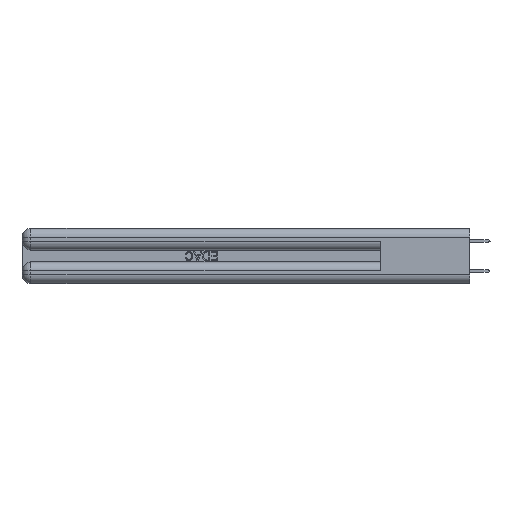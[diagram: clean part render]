
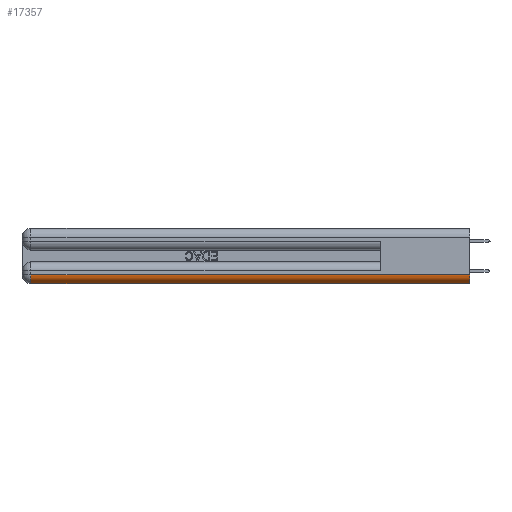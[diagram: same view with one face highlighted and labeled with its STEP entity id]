
A CAD part, left-side view. The second image highlights one B-rep face of the part: STEP entity #17357.
In plain terms, the highlighted cylindrical face has radius 1.524 mm (diameter 3.048 mm), a partial arc.
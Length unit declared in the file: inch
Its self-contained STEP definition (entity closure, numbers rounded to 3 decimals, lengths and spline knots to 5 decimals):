
#22 = CYLINDRICAL_SURFACE ( 'NONE', #30454, 0.06 ) ;
#61 = LINE ( 'NONE', #21087, #33446 ) ;
#102 = AXIS2_PLACEMENT_3D ( 'NONE', #38041, #6338, #45250 ) ;
#2767 = VERTEX_POINT ( 'NONE', #3020 ) ;
#3020 = CARTESIAN_POINT ( 'NONE',  ( 0., 0., 0.06 ) ) ;
#3803 = DIRECTION ( 'NONE',  ( 0., -1., 0. ) ) ;
#6338 = DIRECTION ( 'NONE',  ( 0., 1., 0. ) ) ;
#7774 = CARTESIAN_POINT ( 'NONE',  ( 0.06, 2.94, 0. ) ) ;
#9703 = DIRECTION ( 'NONE',  ( 0., -1., 0. ) ) ;
#9736 = CIRCLE ( 'NONE', #102, 0.06 ) ;
#13907 = DIRECTION ( 'NONE',  ( 0., 0., 1. ) ) ;
#17357 = ADVANCED_FACE ( 'NONE', ( #35016 ), #22, .T. ) ;
#20125 = EDGE_CURVE ( 'NONE', #2767, #30517, #38081, .T. ) ;
#21087 = CARTESIAN_POINT ( 'NONE',  ( 0., 0., 0.06 ) ) ;
#21314 = CARTESIAN_POINT ( 'NONE',  ( 0., 2.94, 0.06 ) ) ;
#23060 = ORIENTED_EDGE ( 'NONE', *, *, #20125, .F. ) ;
#23901 = AXIS2_PLACEMENT_3D ( 'NONE', #42094, #9703, #13907 ) ;
#24977 = CARTESIAN_POINT ( 'NONE',  ( 0.06, 0., 0.06 ) ) ;
#29100 = CARTESIAN_POINT ( 'NONE',  ( 0.06, 0., 0. ) ) ;
#29846 = LINE ( 'NONE', #33559, #37324 ) ;
#30108 = EDGE_CURVE ( 'NONE', #43690, #2767, #61, .T. ) ;
#30454 = AXIS2_PLACEMENT_3D ( 'NONE', #24977, #42917, #31294 ) ;
#30517 = VERTEX_POINT ( 'NONE', #29100 ) ;
#31294 = DIRECTION ( 'NONE',  ( 0., 0., 1. ) ) ;
#31676 = EDGE_CURVE ( 'NONE', #32683, #43690, #9736, .T. ) ;
#31898 = EDGE_CURVE ( 'NONE', #30517, #32683, #29846, .T. ) ;
#32683 = VERTEX_POINT ( 'NONE', #7774 ) ;
#33446 = VECTOR ( 'NONE', #3803, 39.37008 ) ;
#33559 = CARTESIAN_POINT ( 'NONE',  ( 0.06, 3., 0. ) ) ;
#35016 = FACE_OUTER_BOUND ( 'NONE', #36921, .T. ) ;
#35909 = ORIENTED_EDGE ( 'NONE', *, *, #31898, .F. ) ;
#36375 = DIRECTION ( 'NONE',  ( 0., 1., 0. ) ) ;
#36921 = EDGE_LOOP ( 'NONE', ( #23060, #37634, #44501, #35909 ) ) ;
#37324 = VECTOR ( 'NONE', #36375, 39.37008 ) ;
#37634 = ORIENTED_EDGE ( 'NONE', *, *, #30108, .F. ) ;
#38041 = CARTESIAN_POINT ( 'NONE',  ( 0.06, 2.94, 0.06 ) ) ;
#38081 = CIRCLE ( 'NONE', #23901, 0.06 ) ;
#42094 = CARTESIAN_POINT ( 'NONE',  ( 0.06, 0., 0.06 ) ) ;
#42917 = DIRECTION ( 'NONE',  ( 0., 1., 0. ) ) ;
#43690 = VERTEX_POINT ( 'NONE', #21314 ) ;
#44501 = ORIENTED_EDGE ( 'NONE', *, *, #31676, .F. ) ;
#45250 = DIRECTION ( 'NONE',  ( 0., 0., 1. ) ) ;
